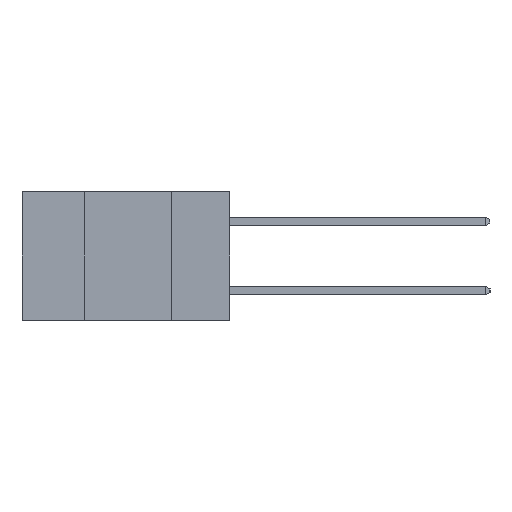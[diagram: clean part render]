
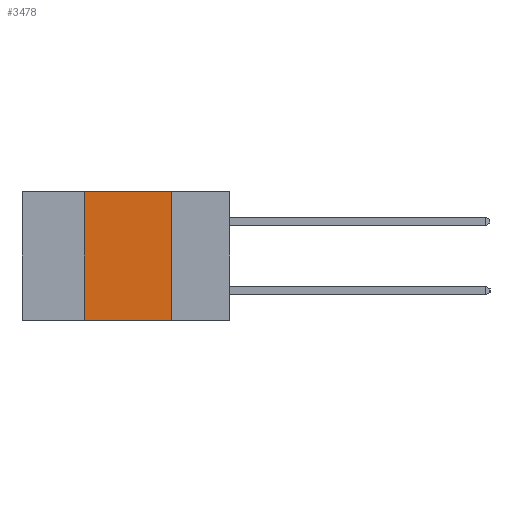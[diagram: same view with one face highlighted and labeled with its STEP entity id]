
A CAD part, left-side view. The second image highlights one B-rep face of the part: STEP entity #3478.
In plain terms, the highlighted planar face has unit normal (-1, 0, 0).
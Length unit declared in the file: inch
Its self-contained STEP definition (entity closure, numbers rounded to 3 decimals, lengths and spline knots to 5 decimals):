
#552 = DIRECTION ( 'NONE',  ( 0., -1., 0. ) ) ;
#720 = VECTOR ( 'NONE', #20053, 39.37008 ) ;
#1851 = VECTOR ( 'NONE', #14837, 39.37008 ) ;
#2639 = CARTESIAN_POINT ( 'NONE',  ( 0., 0.42, -0.37 ) ) ;
#3271 = EDGE_CURVE ( 'NONE', #4419, #17860, #13790, .T. ) ;
#3478 = ADVANCED_FACE ( 'NONE', ( #18780 ), #20809, .F. ) ;
#3840 = CARTESIAN_POINT ( 'NONE',  ( 0., 0.17, -0.37 ) ) ;
#4346 = VERTEX_POINT ( 'NONE', #23176 ) ;
#4419 = VERTEX_POINT ( 'NONE', #17562 ) ;
#5687 = CARTESIAN_POINT ( 'NONE',  ( 0., 0.17, -0.37 ) ) ;
#6925 = EDGE_CURVE ( 'NONE', #4346, #17860, #16195, .T. ) ;
#7728 = DIRECTION ( 'NONE',  ( 0., 0., -1. ) ) ;
#8767 = CARTESIAN_POINT ( 'NONE',  ( 0., 0.6, 0. ) ) ;
#10078 = EDGE_CURVE ( 'NONE', #13051, #4346, #22235, .T. ) ;
#10805 = DIRECTION ( 'NONE',  ( 0., 0., -1. ) ) ;
#11197 = CARTESIAN_POINT ( 'NONE',  ( 0., 0.6, -0.37 ) ) ;
#11669 = AXIS2_PLACEMENT_3D ( 'NONE', #8767, #22774, #10805 ) ;
#12458 = ORIENTED_EDGE ( 'NONE', *, *, #3271, .T. ) ;
#13051 = VERTEX_POINT ( 'NONE', #23197 ) ;
#13431 = ORIENTED_EDGE ( 'NONE', *, *, #18168, .F. ) ;
#13790 = LINE ( 'NONE', #11197, #23123 ) ;
#14104 = CARTESIAN_POINT ( 'NONE',  ( 0., 0.6, 0. ) ) ;
#14714 = ORIENTED_EDGE ( 'NONE', *, *, #10078, .F. ) ;
#14837 = DIRECTION ( 'NONE',  ( 0., 0., 1. ) ) ;
#16195 = LINE ( 'NONE', #5687, #26124 ) ;
#17562 = CARTESIAN_POINT ( 'NONE',  ( 0., 0.42, -0.37 ) ) ;
#17860 = VERTEX_POINT ( 'NONE', #3840 ) ;
#18168 = EDGE_CURVE ( 'NONE', #4419, #13051, #22668, .T. ) ;
#18780 = FACE_OUTER_BOUND ( 'NONE', #25155, .T. ) ;
#20053 = DIRECTION ( 'NONE',  ( 0., -1., 0. ) ) ;
#20809 = PLANE ( 'NONE',  #11669 ) ;
#22235 = LINE ( 'NONE', #14104, #720 ) ;
#22668 = LINE ( 'NONE', #2639, #1851 ) ;
#22774 = DIRECTION ( 'NONE',  ( 1., 0., 0. ) ) ;
#23123 = VECTOR ( 'NONE', #552, 39.37008 ) ;
#23176 = CARTESIAN_POINT ( 'NONE',  ( 0., 0.17, 0. ) ) ;
#23197 = CARTESIAN_POINT ( 'NONE',  ( 0., 0.42, 0. ) ) ;
#25009 = ORIENTED_EDGE ( 'NONE', *, *, #6925, .F. ) ;
#25155 = EDGE_LOOP ( 'NONE', ( #25009, #14714, #13431, #12458 ) ) ;
#26124 = VECTOR ( 'NONE', #7728, 39.37008 ) ;
